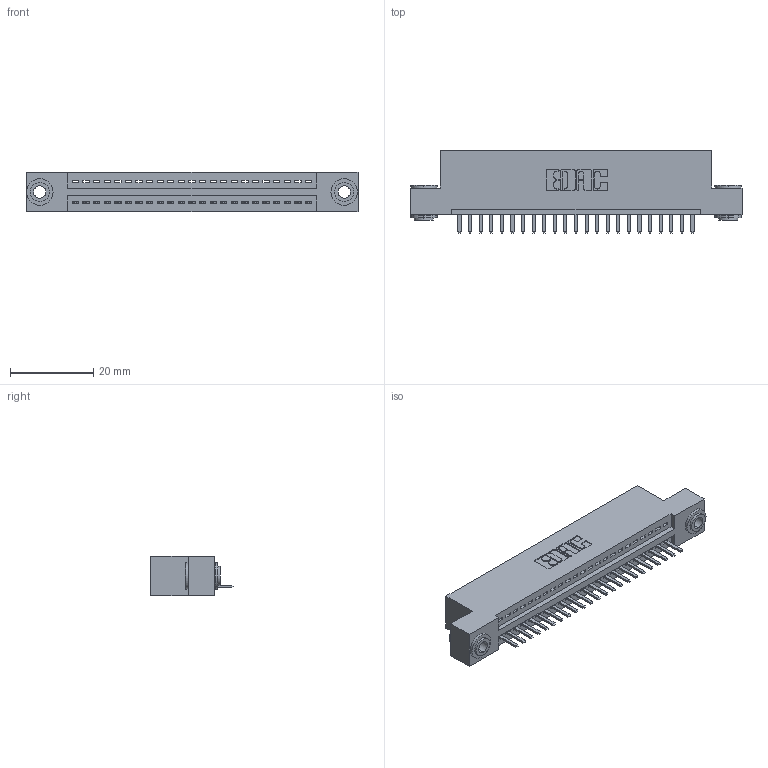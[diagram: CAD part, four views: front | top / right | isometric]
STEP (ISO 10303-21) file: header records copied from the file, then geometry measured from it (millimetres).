
FILE_DESCRIPTION (( 'STEP AP203' ), '1' );
FILE_NAME ('395-023-520-103.STEP', '2019-10-18T03:57:29', ( '' ), ( '' ), 'SwSTEP 2.0', 'SolidWorks 2016', '' );
FILE_SCHEMA (( 'CONFIG_CONTROL_DESIGN' ));
Length unit declared in the file: inch
Products named in the file (4): 345-250-002_345-250-002-102; 395-023-520-103; 345-292-001_345-293-120; 345 Part_Flush Mounting Lugs - 0.156 Dia-TH
Assembly tree (26 placements, depth 2):
  395-023-520-103
    345 Part_Flush Mounting Lugs - 0.156 Dia-TH
    345-292-001_345-293-120  x23
    345-250-002_345-250-002-102  x2
Bounding box: 79.63 x 19.68 x 9.4 mm (x, y, z)
Volume: 7360.8 mm3; surface area: 9521.7 mm2
Topology: 26 solids, 26 shells, 1590 faces, 4649 edges, 3034 vertices
Faces by surface type: plane 1056, cylinder 526, cone 8
Entity records: 20632 total; most frequent: CARTESIAN_POINT 3564, ORIENTED_EDGE 3502, DIRECTION 3159, EDGE_CURVE 1751, VECTOR 1499, LINE 1499, VERTEX_POINT 1162, AXIS2_PLACEMENT_3D 830
